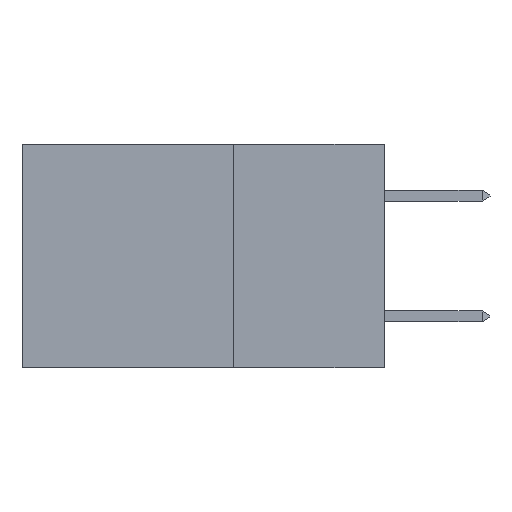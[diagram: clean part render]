
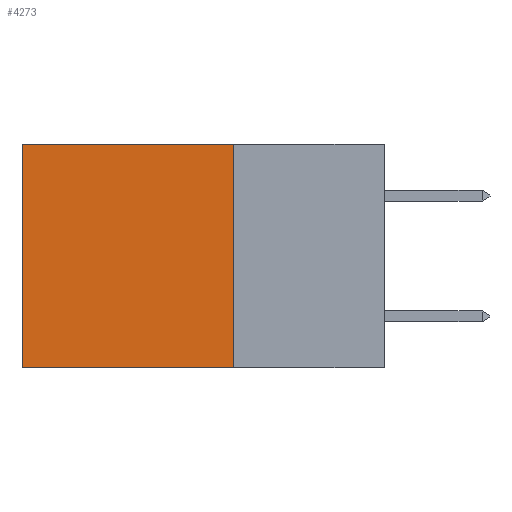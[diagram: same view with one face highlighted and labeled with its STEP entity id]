
A CAD part, left-side view. The second image highlights one B-rep face of the part: STEP entity #4273.
In plain terms, the highlighted planar face has unit normal (-1, 0, 0).
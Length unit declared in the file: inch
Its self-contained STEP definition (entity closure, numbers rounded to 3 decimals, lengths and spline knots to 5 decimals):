
#729 = VECTOR ( 'NONE', #12766, 39.37008 ) ;
#857 = CARTESIAN_POINT ( 'NONE',  ( 0.2875, 0.6, 0. ) ) ;
#896 = EDGE_CURVE ( 'NONE', #12975, #1110, #3655, .T. ) ;
#1110 = VERTEX_POINT ( 'NONE', #2907 ) ;
#1793 = CARTESIAN_POINT ( 'NONE',  ( 0.2875, 0.6, 0. ) ) ;
#1918 = VECTOR ( 'NONE', #4195, 39.37008 ) ;
#2801 = VERTEX_POINT ( 'NONE', #5477 ) ;
#2907 = CARTESIAN_POINT ( 'NONE',  ( 0.2875, 0.6, -0.37 ) ) ;
#2987 = EDGE_LOOP ( 'NONE', ( #10521, #5239, #9614, #8188 ) ) ;
#3655 = LINE ( 'NONE', #6063, #10831 ) ;
#3681 = LINE ( 'NONE', #8585, #4058 ) ;
#4058 = VECTOR ( 'NONE', #7363, 39.37008 ) ;
#4195 = DIRECTION ( 'NONE',  ( 0., 0., -1. ) ) ;
#4273 = ADVANCED_FACE ( 'NONE', ( #4591 ), #5880, .F. ) ;
#4591 = FACE_OUTER_BOUND ( 'NONE', #2987, .T. ) ;
#5239 = ORIENTED_EDGE ( 'NONE', *, *, #896, .F. ) ;
#5403 = CARTESIAN_POINT ( 'NONE',  ( 0.2875, 0.25, 0. ) ) ;
#5477 = CARTESIAN_POINT ( 'NONE',  ( 0.2875, 0.25, 0. ) ) ;
#5742 = AXIS2_PLACEMENT_3D ( 'NONE', #10955, #13298, #12166 ) ;
#5880 = PLANE ( 'NONE',  #5742 ) ;
#6063 = CARTESIAN_POINT ( 'NONE',  ( 0.2875, 0.25, -0.37 ) ) ;
#6848 = EDGE_CURVE ( 'NONE', #2801, #12975, #7888, .T. ) ;
#7363 = DIRECTION ( 'NONE',  ( 0., 1., 0. ) ) ;
#7888 = LINE ( 'NONE', #5403, #1918 ) ;
#8065 = LINE ( 'NONE', #1793, #729 ) ;
#8188 = ORIENTED_EDGE ( 'NONE', *, *, #9650, .T. ) ;
#8303 = CARTESIAN_POINT ( 'NONE',  ( 0.2875, 0.25, -0.37 ) ) ;
#8585 = CARTESIAN_POINT ( 'NONE',  ( 0.2875, 0.25, 0. ) ) ;
#9614 = ORIENTED_EDGE ( 'NONE', *, *, #6848, .F. ) ;
#9650 = EDGE_CURVE ( 'NONE', #2801, #10738, #3681, .T. ) ;
#10521 = ORIENTED_EDGE ( 'NONE', *, *, #12789, .T. ) ;
#10738 = VERTEX_POINT ( 'NONE', #857 ) ;
#10831 = VECTOR ( 'NONE', #10990, 39.37008 ) ;
#10955 = CARTESIAN_POINT ( 'NONE',  ( 0.2875, 0.25, 0. ) ) ;
#10990 = DIRECTION ( 'NONE',  ( 0., 1., 0. ) ) ;
#12166 = DIRECTION ( 'NONE',  ( 0., 0., -1. ) ) ;
#12766 = DIRECTION ( 'NONE',  ( 0., 0., -1. ) ) ;
#12789 = EDGE_CURVE ( 'NONE', #10738, #1110, #8065, .T. ) ;
#12975 = VERTEX_POINT ( 'NONE', #8303 ) ;
#13298 = DIRECTION ( 'NONE',  ( 1., 0., 0. ) ) ;
